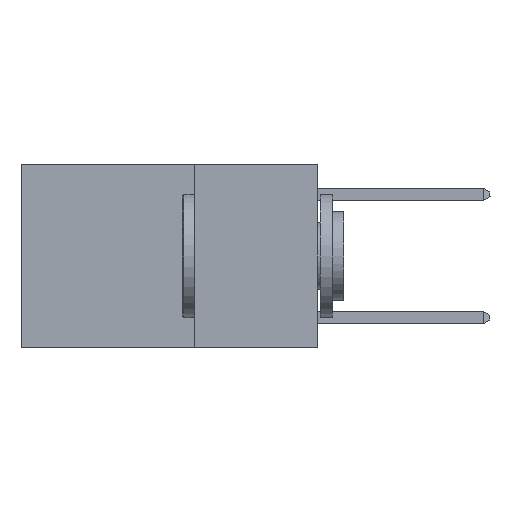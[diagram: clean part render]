
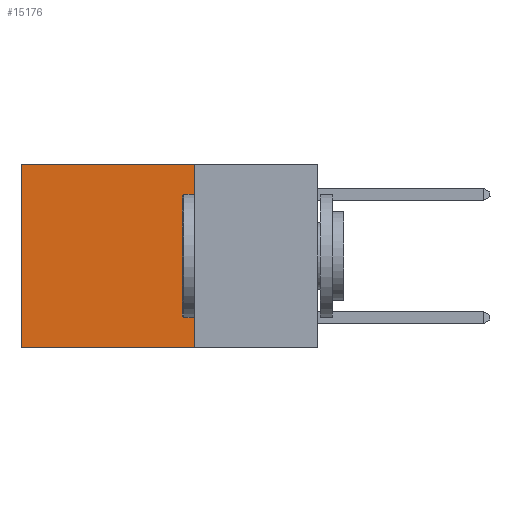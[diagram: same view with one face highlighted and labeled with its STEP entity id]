
A CAD part, left-side view. The second image highlights one B-rep face of the part: STEP entity #15176.
In plain terms, the highlighted planar face has unit normal (-1, 0, 0).
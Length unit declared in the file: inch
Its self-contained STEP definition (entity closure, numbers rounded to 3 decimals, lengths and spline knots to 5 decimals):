
#94 = DIRECTION ( 'NONE',  ( 0., 0., -1. ) ) ;
#668 = CARTESIAN_POINT ( 'NONE',  ( 0.2625, 0.25, -0.37 ) ) ;
#1169 = CARTESIAN_POINT ( 'NONE',  ( 0.2625, 0.25, -0.37 ) ) ;
#1231 = ORIENTED_EDGE ( 'NONE', *, *, #20139, .F. ) ;
#2366 = CARTESIAN_POINT ( 'NONE',  ( 0.2625, 0.25, 0. ) ) ;
#2681 = LINE ( 'NONE', #668, #9455 ) ;
#2693 = EDGE_CURVE ( 'NONE', #16664, #17365, #5628, .T. ) ;
#3544 = VERTEX_POINT ( 'NONE', #1169 ) ;
#3756 = CARTESIAN_POINT ( 'NONE',  ( 0.2625, 0.25, 0. ) ) ;
#4558 = DIRECTION ( 'NONE',  ( 0., 1., 0. ) ) ;
#5533 = CARTESIAN_POINT ( 'NONE',  ( 0.2625, 0.6, 0. ) ) ;
#5628 = LINE ( 'NONE', #3756, #21635 ) ;
#8034 = ORIENTED_EDGE ( 'NONE', *, *, #10301, .T. ) ;
#8189 = ORIENTED_EDGE ( 'NONE', *, *, #2693, .T. ) ;
#9220 = DIRECTION ( 'NONE',  ( 1., 0., 0. ) ) ;
#9455 = VECTOR ( 'NONE', #4558, 39.37008 ) ;
#10301 = EDGE_CURVE ( 'NONE', #17365, #12330, #10977, .T. ) ;
#10977 = LINE ( 'NONE', #5533, #16139 ) ;
#10985 = FACE_OUTER_BOUND ( 'NONE', #22998, .T. ) ;
#10989 = CARTESIAN_POINT ( 'NONE',  ( 0.2625, 0.25, 0. ) ) ;
#12330 = VERTEX_POINT ( 'NONE', #16080 ) ;
#12968 = DIRECTION ( 'NONE',  ( 0., 1., 0. ) ) ;
#13200 = PLANE ( 'NONE',  #17369 ) ;
#15020 = DIRECTION ( 'NONE',  ( 0., 0., -1. ) ) ;
#15176 = ADVANCED_FACE ( 'NONE', ( #10985 ), #13200, .F. ) ;
#15330 = DIRECTION ( 'NONE',  ( 0., 0., -1. ) ) ;
#16080 = CARTESIAN_POINT ( 'NONE',  ( 0.2625, 0.6, -0.37 ) ) ;
#16139 = VECTOR ( 'NONE', #94, 39.37008 ) ;
#16664 = VERTEX_POINT ( 'NONE', #10989 ) ;
#17365 = VERTEX_POINT ( 'NONE', #17869 ) ;
#17369 = AXIS2_PLACEMENT_3D ( 'NONE', #20401, #9220, #15330 ) ;
#17869 = CARTESIAN_POINT ( 'NONE',  ( 0.2625, 0.6, 0. ) ) ;
#18549 = LINE ( 'NONE', #2366, #19287 ) ;
#19287 = VECTOR ( 'NONE', #15020, 39.37008 ) ;
#20139 = EDGE_CURVE ( 'NONE', #3544, #12330, #2681, .T. ) ;
#20401 = CARTESIAN_POINT ( 'NONE',  ( 0.2625, 0.25, 0. ) ) ;
#21520 = EDGE_CURVE ( 'NONE', #16664, #3544, #18549, .T. ) ;
#21635 = VECTOR ( 'NONE', #12968, 39.37008 ) ;
#21823 = ORIENTED_EDGE ( 'NONE', *, *, #21520, .F. ) ;
#22998 = EDGE_LOOP ( 'NONE', ( #8034, #1231, #21823, #8189 ) ) ;
